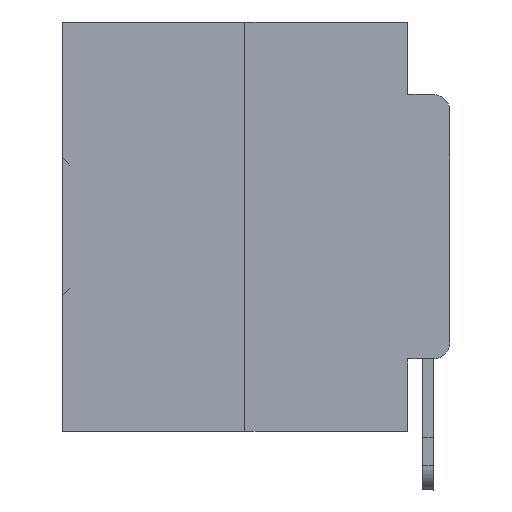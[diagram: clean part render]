
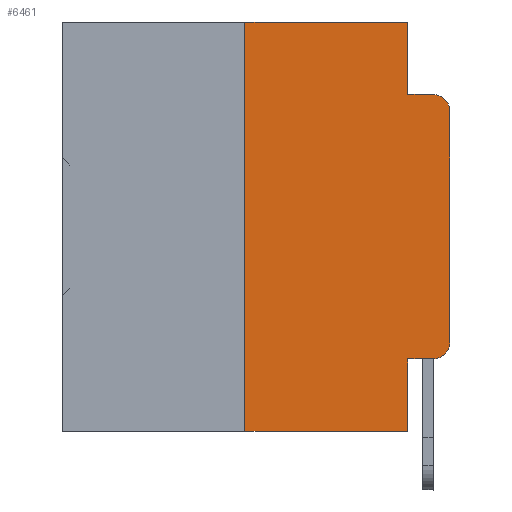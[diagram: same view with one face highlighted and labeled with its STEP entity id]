
A CAD part, left-side view. The second image highlights one B-rep face of the part: STEP entity #6461.
In plain terms, the highlighted planar face has unit normal (-1, 0, 0).
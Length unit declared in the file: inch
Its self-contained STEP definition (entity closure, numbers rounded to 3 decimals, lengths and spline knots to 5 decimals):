
#1027 = LINE ( 'NONE', #35453, #27556 ) ;
#1762 = VECTOR ( 'NONE', #36435, 39.37008 ) ;
#1875 = EDGE_CURVE ( 'NONE', #24294, #6248, #37162, .T. ) ;
#2845 = LINE ( 'NONE', #23082, #7216 ) ;
#2850 = CARTESIAN_POINT ( 'NONE',  ( 0., 0.02, -0.0885 ) ) ;
#3243 = CARTESIAN_POINT ( 'NONE',  ( 0., 0., -0.1085 ) ) ;
#3391 = DIRECTION ( 'NONE',  ( 0., 0., -1. ) ) ;
#3891 = DIRECTION ( 'NONE',  ( 0., 0., -1. ) ) ;
#4104 = CARTESIAN_POINT ( 'NONE',  ( 0., 0.051, -0.0885 ) ) ;
#4581 = LINE ( 'NONE', #5129, #34830 ) ;
#5129 = CARTESIAN_POINT ( 'NONE',  ( 0., 0.473, -0.5 ) ) ;
#5426 = ORIENTED_EDGE ( 'NONE', *, *, #21797, .T. ) ;
#5444 = CARTESIAN_POINT ( 'NONE',  ( 0., 0.051, -0.5 ) ) ;
#5866 = CARTESIAN_POINT ( 'NONE',  ( 0., 0.473, 0. ) ) ;
#5992 = VERTEX_POINT ( 'NONE', #31826 ) ;
#6248 = VERTEX_POINT ( 'NONE', #2850 ) ;
#6312 = AXIS2_PLACEMENT_3D ( 'NONE', #5866, #28957, #17606 ) ;
#6337 = CIRCLE ( 'NONE', #14794, 0.02 ) ;
#6461 = ADVANCED_FACE ( 'NONE', ( #11552 ), #23090, .F. ) ;
#6808 = VERTEX_POINT ( 'NONE', #6892 ) ;
#6817 = VERTEX_POINT ( 'NONE', #15594 ) ;
#6892 = CARTESIAN_POINT ( 'NONE',  ( 0., 0.051, 0. ) ) ;
#7216 = VECTOR ( 'NONE', #17779, 39.37008 ) ;
#7701 = ORIENTED_EDGE ( 'NONE', *, *, #14236, .F. ) ;
#8418 = VECTOR ( 'NONE', #14440, 39.37008 ) ;
#9046 = CARTESIAN_POINT ( 'NONE',  ( 0., 0.051, -0.0885 ) ) ;
#9420 = EDGE_CURVE ( 'NONE', #37061, #18791, #6337, .T. ) ;
#9685 = CARTESIAN_POINT ( 'NONE',  ( 0., 0.02, -0.4115 ) ) ;
#9784 = CARTESIAN_POINT ( 'NONE',  ( 0., 0.02, -0.3915 ) ) ;
#10088 = CARTESIAN_POINT ( 'NONE',  ( 0., 0., -0.3915 ) ) ;
#11073 = VERTEX_POINT ( 'NONE', #5444 ) ;
#11552 = FACE_OUTER_BOUND ( 'NONE', #17174, .T. ) ;
#12085 = CARTESIAN_POINT ( 'NONE',  ( 0., 0.02, -0.1085 ) ) ;
#12805 = EDGE_CURVE ( 'NONE', #20219, #6808, #16205, .T. ) ;
#12941 = CARTESIAN_POINT ( 'NONE',  ( 0., 0.051, 0. ) ) ;
#13090 = DIRECTION ( 'NONE',  ( 0., -1., 0. ) ) ;
#13315 = EDGE_CURVE ( 'NONE', #5992, #20219, #19924, .T. ) ;
#13370 = CARTESIAN_POINT ( 'NONE',  ( 0., 0.473, 0. ) ) ;
#14064 = CARTESIAN_POINT ( 'NONE',  ( 0., 0.25, 0. ) ) ;
#14236 = EDGE_CURVE ( 'NONE', #6817, #11073, #18263, .T. ) ;
#14440 = DIRECTION ( 'NONE',  ( 0., 0., 1. ) ) ;
#14794 = AXIS2_PLACEMENT_3D ( 'NONE', #9784, #18681, #30036 ) ;
#15594 = CARTESIAN_POINT ( 'NONE',  ( 0., 0.051, -0.4115 ) ) ;
#15882 = ORIENTED_EDGE ( 'NONE', *, *, #9420, .T. ) ;
#16205 = LINE ( 'NONE', #13370, #1762 ) ;
#16807 = EDGE_CURVE ( 'NONE', #19542, #6248, #26648, .T. ) ;
#16820 = LINE ( 'NONE', #23066, #20867 ) ;
#17174 = EDGE_LOOP ( 'NONE', ( #37059, #25889, #21312, #24754, #30594, #24952, #5426, #7701, #18660, #15882 ) ) ;
#17606 = DIRECTION ( 'NONE',  ( 0., 0., -1. ) ) ;
#17680 = DIRECTION ( 'NONE',  ( 0., 0., -1. ) ) ;
#17779 = DIRECTION ( 'NONE',  ( 0., -1., 0. ) ) ;
#18263 = LINE ( 'NONE', #12941, #31420 ) ;
#18660 = ORIENTED_EDGE ( 'NONE', *, *, #31351, .T. ) ;
#18681 = DIRECTION ( 'NONE',  ( -1., 0., 0. ) ) ;
#18791 = VERTEX_POINT ( 'NONE', #10088 ) ;
#19542 = VERTEX_POINT ( 'NONE', #4104 ) ;
#19924 = LINE ( 'NONE', #28823, #8418 ) ;
#20219 = VERTEX_POINT ( 'NONE', #14064 ) ;
#20867 = VECTOR ( 'NONE', #34219, 39.37008 ) ;
#21157 = DIRECTION ( 'NONE',  ( 0., -1., 0. ) ) ;
#21312 = ORIENTED_EDGE ( 'NONE', *, *, #16807, .F. ) ;
#21797 = EDGE_CURVE ( 'NONE', #5992, #11073, #4581, .T. ) ;
#23066 = CARTESIAN_POINT ( 'NONE',  ( 0., 0., 0. ) ) ;
#23082 = CARTESIAN_POINT ( 'NONE',  ( 0., 0.051, -0.4115 ) ) ;
#23090 = PLANE ( 'NONE',  #6312 ) ;
#23628 = DIRECTION ( 'NONE',  ( -1., 0., 0. ) ) ;
#24294 = VERTEX_POINT ( 'NONE', #3243 ) ;
#24754 = ORIENTED_EDGE ( 'NONE', *, *, #27623, .F. ) ;
#24952 = ORIENTED_EDGE ( 'NONE', *, *, #13315, .F. ) ;
#25545 = VECTOR ( 'NONE', #21157, 39.37008 ) ;
#25854 = EDGE_CURVE ( 'NONE', #18791, #24294, #16820, .T. ) ;
#25889 = ORIENTED_EDGE ( 'NONE', *, *, #1875, .T. ) ;
#26648 = LINE ( 'NONE', #9046, #25545 ) ;
#27556 = VECTOR ( 'NONE', #17680, 39.37008 ) ;
#27623 = EDGE_CURVE ( 'NONE', #6808, #19542, #1027, .T. ) ;
#28823 = CARTESIAN_POINT ( 'NONE',  ( 0., 0.25, 0. ) ) ;
#28957 = DIRECTION ( 'NONE',  ( 1., 0., 0. ) ) ;
#29326 = AXIS2_PLACEMENT_3D ( 'NONE', #12085, #23628, #3391 ) ;
#30036 = DIRECTION ( 'NONE',  ( 0., 0., -1. ) ) ;
#30594 = ORIENTED_EDGE ( 'NONE', *, *, #12805, .F. ) ;
#31351 = EDGE_CURVE ( 'NONE', #6817, #37061, #2845, .T. ) ;
#31420 = VECTOR ( 'NONE', #3891, 39.37008 ) ;
#31826 = CARTESIAN_POINT ( 'NONE',  ( 0., 0.25, -0.5 ) ) ;
#34219 = DIRECTION ( 'NONE',  ( 0., 0., 1. ) ) ;
#34830 = VECTOR ( 'NONE', #13090, 39.37008 ) ;
#35453 = CARTESIAN_POINT ( 'NONE',  ( 0., 0.051, 0. ) ) ;
#36435 = DIRECTION ( 'NONE',  ( 0., -1., 0. ) ) ;
#37059 = ORIENTED_EDGE ( 'NONE', *, *, #25854, .T. ) ;
#37061 = VERTEX_POINT ( 'NONE', #9685 ) ;
#37162 = CIRCLE ( 'NONE', #29326, 0.02 ) ;
